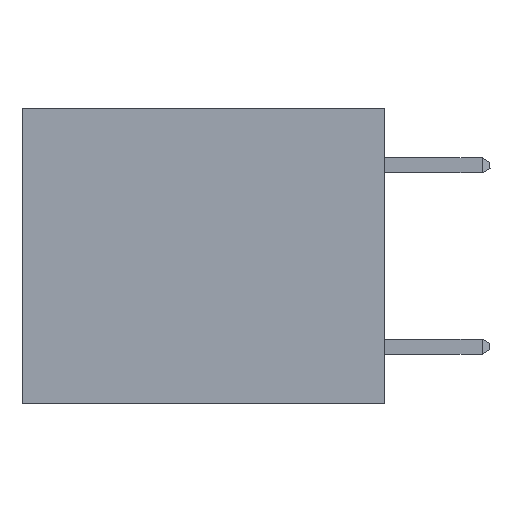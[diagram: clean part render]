
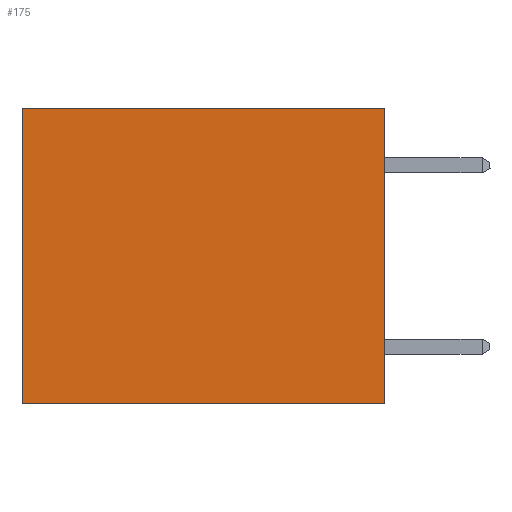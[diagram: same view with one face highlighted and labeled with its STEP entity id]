
A CAD part, left-side view. The second image highlights one B-rep face of the part: STEP entity #175.
In plain terms, the highlighted planar face has unit normal (-1, 0, 0).
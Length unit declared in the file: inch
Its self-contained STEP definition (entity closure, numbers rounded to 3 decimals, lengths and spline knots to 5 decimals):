
#175 = ADVANCED_FACE ( 'NONE', ( #6539 ), #817, .F. ) ;
#817 = PLANE ( 'NONE',  #19699 ) ;
#877 = DIRECTION ( 'NONE',  ( 0., 1., 0. ) ) ;
#980 = VECTOR ( 'NONE', #2378, 39.37008 ) ;
#2378 = DIRECTION ( 'NONE',  ( 0., 0., -1. ) ) ;
#2608 = CARTESIAN_POINT ( 'NONE',  ( 0.3165, 0., -0.49 ) ) ;
#3318 = LINE ( 'NONE', #5835, #4080 ) ;
#4080 = VECTOR ( 'NONE', #17930, 39.37008 ) ;
#5171 = EDGE_CURVE ( 'NONE', #19809, #13635, #5498, .T. ) ;
#5498 = LINE ( 'NONE', #8695, #980 ) ;
#5736 = ORIENTED_EDGE ( 'NONE', *, *, #12947, .F. ) ;
#5835 = CARTESIAN_POINT ( 'NONE',  ( 0.3165, 0., 0. ) ) ;
#6539 = FACE_OUTER_BOUND ( 'NONE', #19208, .T. ) ;
#7246 = EDGE_CURVE ( 'NONE', #7849, #19809, #3318, .T. ) ;
#7849 = VERTEX_POINT ( 'NONE', #14994 ) ;
#8635 = ORIENTED_EDGE ( 'NONE', *, *, #5171, .T. ) ;
#8695 = CARTESIAN_POINT ( 'NONE',  ( 0.3165, 0.6, -0.49 ) ) ;
#9274 = CARTESIAN_POINT ( 'NONE',  ( 0.3165, 0., -0.49 ) ) ;
#9475 = CARTESIAN_POINT ( 'NONE',  ( 0.3165, 0., -0.49 ) ) ;
#10649 = CARTESIAN_POINT ( 'NONE',  ( 0.3165, 0., -0.49 ) ) ;
#12947 = EDGE_CURVE ( 'NONE', #22069, #13635, #17848, .T. ) ;
#13360 = ORIENTED_EDGE ( 'NONE', *, *, #14801, .F. ) ;
#13635 = VERTEX_POINT ( 'NONE', #17658 ) ;
#13993 = VECTOR ( 'NONE', #15824, 39.37008 ) ;
#14801 = EDGE_CURVE ( 'NONE', #7849, #22069, #18015, .T. ) ;
#14994 = CARTESIAN_POINT ( 'NONE',  ( 0.3165, 0., 0. ) ) ;
#15643 = ORIENTED_EDGE ( 'NONE', *, *, #7246, .T. ) ;
#15824 = DIRECTION ( 'NONE',  ( 0., 0., -1. ) ) ;
#16037 = DIRECTION ( 'NONE',  ( 0., 0., -1. ) ) ;
#16103 = DIRECTION ( 'NONE',  ( 1., 0., 0. ) ) ;
#16783 = VECTOR ( 'NONE', #877, 39.37008 ) ;
#17658 = CARTESIAN_POINT ( 'NONE',  ( 0.3165, 0.6, -0.49 ) ) ;
#17848 = LINE ( 'NONE', #9475, #16783 ) ;
#17930 = DIRECTION ( 'NONE',  ( 0., 1., 0. ) ) ;
#18015 = LINE ( 'NONE', #10649, #13993 ) ;
#19208 = EDGE_LOOP ( 'NONE', ( #8635, #5736, #13360, #15643 ) ) ;
#19699 = AXIS2_PLACEMENT_3D ( 'NONE', #9274, #16103, #16037 ) ;
#19809 = VERTEX_POINT ( 'NONE', #19831 ) ;
#19831 = CARTESIAN_POINT ( 'NONE',  ( 0.3165, 0.6, 0. ) ) ;
#22069 = VERTEX_POINT ( 'NONE', #2608 ) ;
